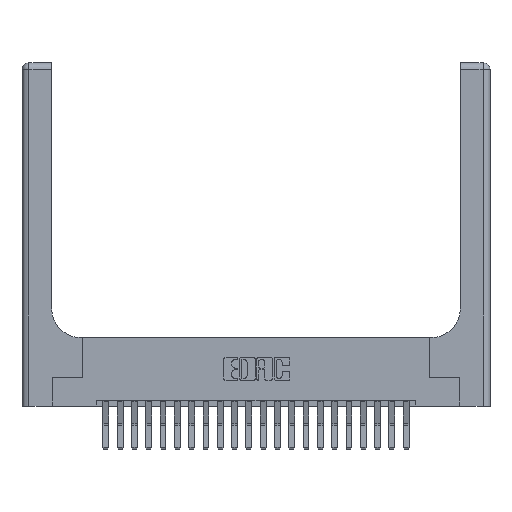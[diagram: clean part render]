
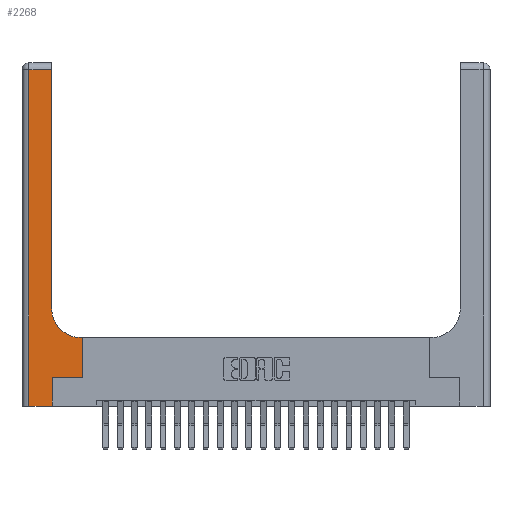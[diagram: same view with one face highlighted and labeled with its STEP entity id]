
A CAD part, top view. The second image highlights one B-rep face of the part: STEP entity #2268.
In plain terms, the highlighted planar face has unit normal (0, 0, 1).
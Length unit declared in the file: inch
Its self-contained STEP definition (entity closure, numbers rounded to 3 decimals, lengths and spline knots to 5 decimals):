
#406 = CARTESIAN_POINT ( 'NONE',  ( 0.26, 3., 0.37 ) ) ;
#475 = VECTOR ( 'NONE', #2927, 39.37008 ) ;
#576 = DIRECTION ( 'NONE',  ( 1., 0., 0. ) ) ;
#1160 = VERTEX_POINT ( 'NONE', #15970 ) ;
#1590 = CARTESIAN_POINT ( 'NONE',  ( 0.265, 0., 0.37 ) ) ;
#1753 = EDGE_CURVE ( 'NONE', #20146, #8537, #7573, .T. ) ;
#2160 = DIRECTION ( 'NONE',  ( 0., 1., 0. ) ) ;
#2268 = ADVANCED_FACE ( 'NONE', ( #21342 ), #8428, .F. ) ;
#2312 = DIRECTION ( 'NONE',  ( 1., 0., 0. ) ) ;
#2719 = LINE ( 'NONE', #3919, #20519 ) ;
#2927 = DIRECTION ( 'NONE',  ( 0., -1., 0. ) ) ;
#2982 = DIRECTION ( 'NONE',  ( 1., 0., 0. ) ) ;
#3137 = EDGE_CURVE ( 'NONE', #18449, #1160, #15896, .T. ) ;
#3317 = DIRECTION ( 'NONE',  ( 0., 1., 0. ) ) ;
#3871 = VERTEX_POINT ( 'NONE', #6493 ) ;
#3919 = CARTESIAN_POINT ( 'NONE',  ( 0., 0., 0.37 ) ) ;
#4111 = VECTOR ( 'NONE', #2982, 39.37008 ) ;
#4797 = LINE ( 'NONE', #9698, #475 ) ;
#5586 = DIRECTION ( 'NONE',  ( 0., 0., -1. ) ) ;
#6372 = EDGE_CURVE ( 'NONE', #7429, #3871, #2719, .T. ) ;
#6493 = CARTESIAN_POINT ( 'NONE',  ( 0.265, 0., 0.37 ) ) ;
#6527 = CARTESIAN_POINT ( 'NONE',  ( 0.06, 2.94, 0.37 ) ) ;
#6660 = AXIS2_PLACEMENT_3D ( 'NONE', #20523, #11624, #22250 ) ;
#7429 = VERTEX_POINT ( 'NONE', #17009 ) ;
#7573 = LINE ( 'NONE', #18600, #4111 ) ;
#8306 = LINE ( 'NONE', #20560, #16920 ) ;
#8428 = PLANE ( 'NONE',  #6660 ) ;
#8537 = VERTEX_POINT ( 'NONE', #10766 ) ;
#8580 = ORIENTED_EDGE ( 'NONE', *, *, #13724, .T. ) ;
#9698 = CARTESIAN_POINT ( 'NONE',  ( 0.06, 3., 0.37 ) ) ;
#9975 = CARTESIAN_POINT ( 'NONE',  ( 0.528, 0.6, 0.37 ) ) ;
#10456 = LINE ( 'NONE', #19362, #19371 ) ;
#10484 = VECTOR ( 'NONE', #3317, 39.37008 ) ;
#10721 = EDGE_CURVE ( 'NONE', #1160, #15141, #15705, .T. ) ;
#10766 = CARTESIAN_POINT ( 'NONE',  ( 0.528, 0.25, 0.37 ) ) ;
#11178 = LINE ( 'NONE', #17095, #18728 ) ;
#11239 = CARTESIAN_POINT ( 'NONE',  ( 0.26, 2.94, 0.37 ) ) ;
#11624 = DIRECTION ( 'NONE',  ( 0., 0., -1. ) ) ;
#12123 = LINE ( 'NONE', #1590, #10484 ) ;
#12486 = DIRECTION ( 'NONE',  ( -1., 0., 0. ) ) ;
#12625 = CARTESIAN_POINT ( 'NONE',  ( 0.51, 0.85, 0.37 ) ) ;
#13037 = CARTESIAN_POINT ( 'NONE',  ( 0.265, 0.25, 0.37 ) ) ;
#13130 = EDGE_CURVE ( 'NONE', #3871, #20146, #12123, .T. ) ;
#13341 = CARTESIAN_POINT ( 'NONE',  ( 0.51, 0.6, 0.37 ) ) ;
#13427 = DIRECTION ( 'NONE',  ( 0., 1., 0. ) ) ;
#13582 = ORIENTED_EDGE ( 'NONE', *, *, #19128, .T. ) ;
#13724 = EDGE_CURVE ( 'NONE', #15141, #16484, #10456, .T. ) ;
#14732 = ORIENTED_EDGE ( 'NONE', *, *, #1753, .T. ) ;
#15097 = AXIS2_PLACEMENT_3D ( 'NONE', #12625, #5586, #2312 ) ;
#15141 = VERTEX_POINT ( 'NONE', #11239 ) ;
#15705 = LINE ( 'NONE', #406, #17323 ) ;
#15896 = CIRCLE ( 'NONE', #15097, 0.25 ) ;
#15970 = CARTESIAN_POINT ( 'NONE',  ( 0.26, 0.85, 0.37 ) ) ;
#16397 = ORIENTED_EDGE ( 'NONE', *, *, #10721, .T. ) ;
#16484 = VERTEX_POINT ( 'NONE', #6527 ) ;
#16691 = ORIENTED_EDGE ( 'NONE', *, *, #13130, .T. ) ;
#16920 = VECTOR ( 'NONE', #17050, 39.37008 ) ;
#17009 = CARTESIAN_POINT ( 'NONE',  ( 0.06, 0., 0.37 ) ) ;
#17050 = DIRECTION ( 'NONE',  ( -1., 0., 0. ) ) ;
#17095 = CARTESIAN_POINT ( 'NONE',  ( 0.528, 0.25, 0.37 ) ) ;
#17323 = VECTOR ( 'NONE', #2160, 39.37008 ) ;
#17570 = EDGE_CURVE ( 'NONE', #8537, #20906, #11178, .T. ) ;
#17600 = ORIENTED_EDGE ( 'NONE', *, *, #20280, .T. ) ;
#18449 = VERTEX_POINT ( 'NONE', #13341 ) ;
#18600 = CARTESIAN_POINT ( 'NONE',  ( 0.265, 0.25, 0.37 ) ) ;
#18711 = ORIENTED_EDGE ( 'NONE', *, *, #6372, .T. ) ;
#18728 = VECTOR ( 'NONE', #13427, 39.37008 ) ;
#19128 = EDGE_CURVE ( 'NONE', #20906, #18449, #8306, .T. ) ;
#19362 = CARTESIAN_POINT ( 'NONE',  ( 0., 2.94, 0.37 ) ) ;
#19371 = VECTOR ( 'NONE', #12486, 39.37008 ) ;
#20146 = VERTEX_POINT ( 'NONE', #13037 ) ;
#20280 = EDGE_CURVE ( 'NONE', #16484, #7429, #4797, .T. ) ;
#20519 = VECTOR ( 'NONE', #576, 39.37008 ) ;
#20523 = CARTESIAN_POINT ( 'NONE',  ( 0., 3., 0.37 ) ) ;
#20560 = CARTESIAN_POINT ( 'NONE',  ( 0.26, 0.6, 0.37 ) ) ;
#20662 = EDGE_LOOP ( 'NONE', ( #16397, #8580, #17600, #18711, #16691, #14732, #21525, #13582, #20681 ) ) ;
#20681 = ORIENTED_EDGE ( 'NONE', *, *, #3137, .T. ) ;
#20906 = VERTEX_POINT ( 'NONE', #9975 ) ;
#21342 = FACE_OUTER_BOUND ( 'NONE', #20662, .T. ) ;
#21525 = ORIENTED_EDGE ( 'NONE', *, *, #17570, .T. ) ;
#22250 = DIRECTION ( 'NONE',  ( -1., 0., 0. ) ) ;
